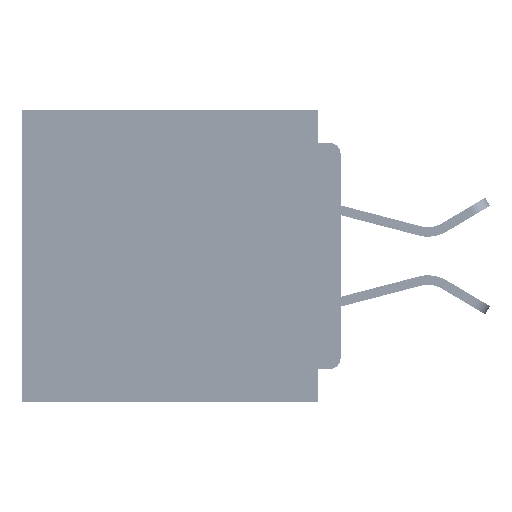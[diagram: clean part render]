
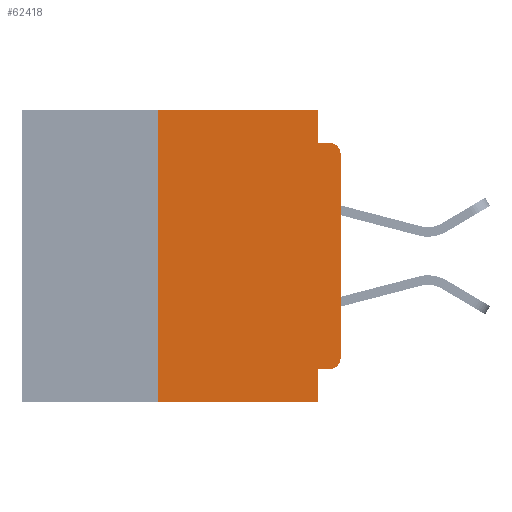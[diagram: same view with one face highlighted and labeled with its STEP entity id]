
A CAD part, left-side view. The second image highlights one B-rep face of the part: STEP entity #62418.
In plain terms, the highlighted planar face has unit normal (-1, 0, 0).
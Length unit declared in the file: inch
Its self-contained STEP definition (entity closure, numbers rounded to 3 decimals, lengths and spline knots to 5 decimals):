
#94 = CARTESIAN_POINT ( 'NONE',  ( 0., 0., -0.06 ) ) ;
#218 = VERTEX_POINT ( 'NONE', #36935 ) ;
#3657 = CARTESIAN_POINT ( 'NONE',  ( 0., 0., -0.355 ) ) ;
#3660 = CARTESIAN_POINT ( 'NONE',  ( 0., 0.031, -0.4 ) ) ;
#4505 = ORIENTED_EDGE ( 'NONE', *, *, #15026, .F. ) ;
#4986 = EDGE_CURVE ( 'NONE', #30692, #57218, #31974, .T. ) ;
#5279 = CARTESIAN_POINT ( 'NONE',  ( 0., 0.031, 0. ) ) ;
#6510 = CARTESIAN_POINT ( 'NONE',  ( 0., 0.25, -0.4 ) ) ;
#8151 = VECTOR ( 'NONE', #63075, 39.37008 ) ;
#8661 = DIRECTION ( 'NONE',  ( 0., 1., 0. ) ) ;
#8898 = DIRECTION ( 'NONE',  ( 0., 0., -1. ) ) ;
#9796 = LINE ( 'NONE', #6510, #8151 ) ;
#9921 = ORIENTED_EDGE ( 'NONE', *, *, #35191, .F. ) ;
#10415 = CARTESIAN_POINT ( 'NONE',  ( 0., 0.437, -0.4 ) ) ;
#10495 = DIRECTION ( 'NONE',  ( 0., 0., -1. ) ) ;
#11295 = CARTESIAN_POINT ( 'NONE',  ( 0., 0.015, -0.34 ) ) ;
#11644 = CARTESIAN_POINT ( 'NONE',  ( 0., 0.015, -0.06 ) ) ;
#11940 = CARTESIAN_POINT ( 'NONE',  ( 0., 0., 0. ) ) ;
#12205 = VECTOR ( 'NONE', #8898, 39.37008 ) ;
#13329 = ORIENTED_EDGE ( 'NONE', *, *, #29681, .F. ) ;
#14032 = EDGE_CURVE ( 'NONE', #218, #30692, #41779, .T. ) ;
#14774 = DIRECTION ( 'NONE',  ( 0., 0., -1. ) ) ;
#15026 = EDGE_CURVE ( 'NONE', #218, #23357, #48838, .T. ) ;
#15501 = EDGE_LOOP ( 'NONE', ( #21099, #31177, #55764, #9921, #13329, #62895, #29903, #39858, #4505, #17802 ) ) ;
#16499 = VECTOR ( 'NONE', #10495, 39.37008 ) ;
#16520 = DIRECTION ( 'NONE',  ( 0., 0., -1. ) ) ;
#16711 = VERTEX_POINT ( 'NONE', #55710 ) ;
#16865 = DIRECTION ( 'NONE',  ( 0., 0., -1. ) ) ;
#17278 = EDGE_CURVE ( 'NONE', #23357, #66036, #27623, .T. ) ;
#17802 = ORIENTED_EDGE ( 'NONE', *, *, #14032, .T. ) ;
#18125 = LINE ( 'NONE', #5279, #16499 ) ;
#19724 = AXIS2_PLACEMENT_3D ( 'NONE', #11644, #47810, #16865 ) ;
#20723 = LINE ( 'NONE', #10415, #46590 ) ;
#20749 = CIRCLE ( 'NONE', #19724, 0.015 ) ;
#20772 = FACE_OUTER_BOUND ( 'NONE', #15501, .T. ) ;
#21099 = ORIENTED_EDGE ( 'NONE', *, *, #4986, .T. ) ;
#21437 = EDGE_CURVE ( 'NONE', #60644, #66036, #20723, .T. ) ;
#22098 = VERTEX_POINT ( 'NONE', #62378 ) ;
#22411 = LINE ( 'NONE', #66075, #60250 ) ;
#23186 = VERTEX_POINT ( 'NONE', #51344 ) ;
#23357 = VERTEX_POINT ( 'NONE', #42596 ) ;
#23801 = DIRECTION ( 'NONE',  ( 0., -1., 0. ) ) ;
#27516 = VECTOR ( 'NONE', #23801, 39.37008 ) ;
#27623 = LINE ( 'NONE', #3660, #12205 ) ;
#28312 = EDGE_CURVE ( 'NONE', #22098, #23186, #63622, .T. ) ;
#28514 = VERTEX_POINT ( 'NONE', #57157 ) ;
#28838 = CARTESIAN_POINT ( 'NONE',  ( 0., 0., -0.045 ) ) ;
#29681 = EDGE_CURVE ( 'NONE', #16711, #28514, #22411, .T. ) ;
#29903 = ORIENTED_EDGE ( 'NONE', *, *, #21437, .T. ) ;
#30692 = VERTEX_POINT ( 'NONE', #40047 ) ;
#31177 = ORIENTED_EDGE ( 'NONE', *, *, #41070, .T. ) ;
#31974 = LINE ( 'NONE', #11940, #57687 ) ;
#35191 = EDGE_CURVE ( 'NONE', #28514, #22098, #18125, .T. ) ;
#35472 = DIRECTION ( 'NONE',  ( 0., -1., 0. ) ) ;
#36277 = DIRECTION ( 'NONE',  ( 0., -1., 0. ) ) ;
#36935 = CARTESIAN_POINT ( 'NONE',  ( 0., 0.015, -0.355 ) ) ;
#37888 = AXIS2_PLACEMENT_3D ( 'NONE', #11295, #47465, #16520 ) ;
#39858 = ORIENTED_EDGE ( 'NONE', *, *, #17278, .F. ) ;
#40047 = CARTESIAN_POINT ( 'NONE',  ( 0., 0., -0.34 ) ) ;
#40638 = PLANE ( 'NONE',  #53815 ) ;
#41070 = EDGE_CURVE ( 'NONE', #57218, #23186, #20749, .T. ) ;
#41779 = CIRCLE ( 'NONE', #37888, 0.015 ) ;
#42596 = CARTESIAN_POINT ( 'NONE',  ( 0., 0.031, -0.355 ) ) ;
#42972 = DIRECTION ( 'NONE',  ( 0., 0., 1. ) ) ;
#44328 = CARTESIAN_POINT ( 'NONE',  ( 0., 0.25, -0.4 ) ) ;
#45754 = DIRECTION ( 'NONE',  ( 1., 0., 0. ) ) ;
#46590 = VECTOR ( 'NONE', #36277, 39.37008 ) ;
#47465 = DIRECTION ( 'NONE',  ( -1., 0., 0. ) ) ;
#47810 = DIRECTION ( 'NONE',  ( -1., 0., 0. ) ) ;
#48838 = LINE ( 'NONE', #3657, #59210 ) ;
#51344 = CARTESIAN_POINT ( 'NONE',  ( 0., 0.015, -0.045 ) ) ;
#53815 = AXIS2_PLACEMENT_3D ( 'NONE', #65996, #45754, #14774 ) ;
#55710 = CARTESIAN_POINT ( 'NONE',  ( 0., 0.25, 0. ) ) ;
#55764 = ORIENTED_EDGE ( 'NONE', *, *, #28312, .F. ) ;
#57157 = CARTESIAN_POINT ( 'NONE',  ( 0., 0.031, 0. ) ) ;
#57218 = VERTEX_POINT ( 'NONE', #94 ) ;
#57687 = VECTOR ( 'NONE', #42972, 39.37008 ) ;
#59210 = VECTOR ( 'NONE', #8661, 39.37008 ) ;
#60250 = VECTOR ( 'NONE', #35472, 39.37008 ) ;
#60644 = VERTEX_POINT ( 'NONE', #44328 ) ;
#62378 = CARTESIAN_POINT ( 'NONE',  ( 0., 0.031, -0.045 ) ) ;
#62418 = ADVANCED_FACE ( 'NONE', ( #20772 ), #40638, .F. ) ;
#62895 = ORIENTED_EDGE ( 'NONE', *, *, #65337, .F. ) ;
#63075 = DIRECTION ( 'NONE',  ( 0., 0., 1. ) ) ;
#63423 = CARTESIAN_POINT ( 'NONE',  ( 0., 0.031, -0.4 ) ) ;
#63622 = LINE ( 'NONE', #28838, #27516 ) ;
#65337 = EDGE_CURVE ( 'NONE', #60644, #16711, #9796, .T. ) ;
#65996 = CARTESIAN_POINT ( 'NONE',  ( 0., 0.437, 0. ) ) ;
#66036 = VERTEX_POINT ( 'NONE', #63423 ) ;
#66075 = CARTESIAN_POINT ( 'NONE',  ( 0., 0.437, 0. ) ) ;
